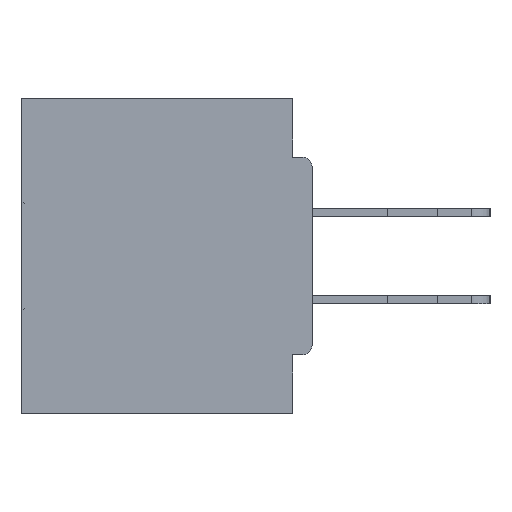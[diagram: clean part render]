
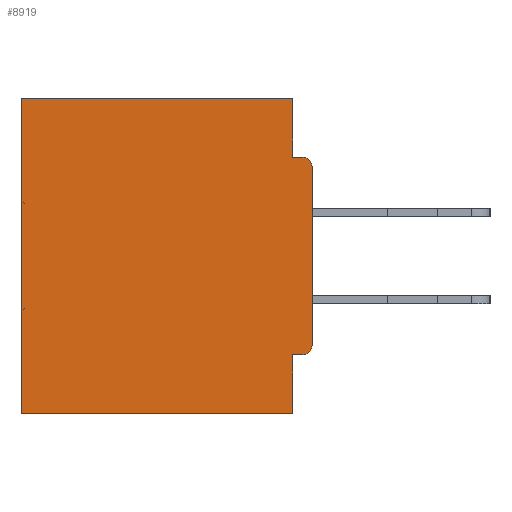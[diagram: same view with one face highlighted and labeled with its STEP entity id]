
A CAD part, left-side view. The second image highlights one B-rep face of the part: STEP entity #8919.
In plain terms, the highlighted planar face has unit normal (-1, 0, 0).
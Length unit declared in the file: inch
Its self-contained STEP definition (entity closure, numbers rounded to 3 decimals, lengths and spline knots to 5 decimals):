
#86 = DIRECTION ( 'NONE',  ( 0., 0., -1. ) ) ;
#171 = VERTEX_POINT ( 'NONE', #35271 ) ;
#204 = CARTESIAN_POINT ( 'NONE',  ( 0.298, 0.031, -0.5 ) ) ;
#538 = PLANE ( 'NONE',  #35679 ) ;
#1322 = EDGE_CURVE ( 'NONE', #26127, #38626, #14939, .T. ) ;
#1695 = CARTESIAN_POINT ( 'NONE',  ( 0.298, 0.015, -0.3915 ) ) ;
#2150 = CARTESIAN_POINT ( 'NONE',  ( 0.298, 0.015, -0.4065 ) ) ;
#3239 = CARTESIAN_POINT ( 'NONE',  ( 0.298, 0.031, -0.5 ) ) ;
#3848 = ORIENTED_EDGE ( 'NONE', *, *, #26362, .T. ) ;
#5564 = VERTEX_POINT ( 'NONE', #32588 ) ;
#6024 = CIRCLE ( 'NONE', #27586, 0.015 ) ;
#6758 = LINE ( 'NONE', #42754, #42551 ) ;
#7148 = ORIENTED_EDGE ( 'NONE', *, *, #35621, .F. ) ;
#7418 = DIRECTION ( 'NONE',  ( 0., 1., 0. ) ) ;
#8202 = VECTOR ( 'NONE', #37123, 39.37008 ) ;
#8390 = EDGE_CURVE ( 'NONE', #37002, #37179, #33414, .T. ) ;
#8805 = EDGE_LOOP ( 'NONE', ( #33632, #7148, #31541, #28815, #23127, #18778, #42385, #15322, #3848, #39202 ) ) ;
#8919 = ADVANCED_FACE ( 'NONE', ( #35030 ), #538, .F. ) ;
#9621 = VECTOR ( 'NONE', #30641, 39.37008 ) ;
#9954 = CARTESIAN_POINT ( 'NONE',  ( 0.298, 0.031, -0.5 ) ) ;
#10310 = CARTESIAN_POINT ( 'NONE',  ( 0.298, 0.031, -0.0935 ) ) ;
#10356 = CARTESIAN_POINT ( 'NONE',  ( 0.298, 0., 0. ) ) ;
#11106 = DIRECTION ( 'NONE',  ( 0., 0., -1. ) ) ;
#11273 = DIRECTION ( 'NONE',  ( 0., 1., 0. ) ) ;
#12420 = CARTESIAN_POINT ( 'NONE',  ( 0.298, 0., -0.3915 ) ) ;
#14620 = LINE ( 'NONE', #20014, #8202 ) ;
#14939 = CIRCLE ( 'NONE', #15940, 0.015 ) ;
#15322 = ORIENTED_EDGE ( 'NONE', *, *, #8390, .F. ) ;
#15940 = AXIS2_PLACEMENT_3D ( 'NONE', #19607, #43459, #26461 ) ;
#17151 = VECTOR ( 'NONE', #86, 39.37008 ) ;
#17632 = VECTOR ( 'NONE', #26953, 39.37008 ) ;
#17995 = CARTESIAN_POINT ( 'NONE',  ( 0.298, 0.031, 0. ) ) ;
#18615 = DIRECTION ( 'NONE',  ( 0., 0., -1. ) ) ;
#18778 = ORIENTED_EDGE ( 'NONE', *, *, #43936, .F. ) ;
#19500 = CARTESIAN_POINT ( 'NONE',  ( 0.298, 0., 0. ) ) ;
#19607 = CARTESIAN_POINT ( 'NONE',  ( 0.298, 0.015, -0.1085 ) ) ;
#20014 = CARTESIAN_POINT ( 'NONE',  ( 0.298, 0., -0.0935 ) ) ;
#20282 = LINE ( 'NONE', #19500, #17632 ) ;
#20614 = CARTESIAN_POINT ( 'NONE',  ( 0.298, 0., -0.5 ) ) ;
#20623 = EDGE_CURVE ( 'NONE', #26127, #36094, #25227, .T. ) ;
#21669 = EDGE_CURVE ( 'NONE', #33006, #5564, #20282, .T. ) ;
#22375 = DIRECTION ( 'NONE',  ( 0., 0., -1. ) ) ;
#23127 = ORIENTED_EDGE ( 'NONE', *, *, #39324, .T. ) ;
#23148 = LINE ( 'NONE', #20614, #28991 ) ;
#23327 = CARTESIAN_POINT ( 'NONE',  ( 0.298, 0., 0. ) ) ;
#25227 = LINE ( 'NONE', #23327, #40081 ) ;
#26127 = VERTEX_POINT ( 'NONE', #34726 ) ;
#26362 = EDGE_CURVE ( 'NONE', #37002, #36094, #6024, .T. ) ;
#26461 = DIRECTION ( 'NONE',  ( 0., 0., -1. ) ) ;
#26953 = DIRECTION ( 'NONE',  ( 0., 1., 0. ) ) ;
#27586 = AXIS2_PLACEMENT_3D ( 'NONE', #1695, #39011, #18615 ) ;
#28815 = ORIENTED_EDGE ( 'NONE', *, *, #21669, .T. ) ;
#28991 = VECTOR ( 'NONE', #7418, 39.37008 ) ;
#29258 = VERTEX_POINT ( 'NONE', #3239 ) ;
#29342 = CARTESIAN_POINT ( 'NONE',  ( 0.298, 0.015, -0.0935 ) ) ;
#30641 = DIRECTION ( 'NONE',  ( 0., 0., -1. ) ) ;
#31358 = EDGE_CURVE ( 'NONE', #37179, #29258, #32598, .T. ) ;
#31519 = CARTESIAN_POINT ( 'NONE',  ( 0.298, 0.031, -0.4065 ) ) ;
#31541 = ORIENTED_EDGE ( 'NONE', *, *, #36929, .F. ) ;
#32588 = CARTESIAN_POINT ( 'NONE',  ( 0.298, 0.46, 0. ) ) ;
#32598 = LINE ( 'NONE', #204, #9621 ) ;
#33006 = VERTEX_POINT ( 'NONE', #17995 ) ;
#33414 = LINE ( 'NONE', #34690, #43570 ) ;
#33632 = ORIENTED_EDGE ( 'NONE', *, *, #1322, .T. ) ;
#34690 = CARTESIAN_POINT ( 'NONE',  ( 0.298, 0., -0.4065 ) ) ;
#34726 = CARTESIAN_POINT ( 'NONE',  ( 0.298, 0., -0.1085 ) ) ;
#34829 = DIRECTION ( 'NONE',  ( 1., 0., 0. ) ) ;
#35030 = FACE_OUTER_BOUND ( 'NONE', #8805, .T. ) ;
#35271 = CARTESIAN_POINT ( 'NONE',  ( 0.298, 0.46, -0.5 ) ) ;
#35621 = EDGE_CURVE ( 'NONE', #42707, #38626, #14620, .T. ) ;
#35679 = AXIS2_PLACEMENT_3D ( 'NONE', #10356, #34829, #11106 ) ;
#36094 = VERTEX_POINT ( 'NONE', #12420 ) ;
#36929 = EDGE_CURVE ( 'NONE', #33006, #42707, #42790, .T. ) ;
#37002 = VERTEX_POINT ( 'NONE', #2150 ) ;
#37123 = DIRECTION ( 'NONE',  ( 0., -1., 0. ) ) ;
#37179 = VERTEX_POINT ( 'NONE', #31519 ) ;
#38626 = VERTEX_POINT ( 'NONE', #29342 ) ;
#39011 = DIRECTION ( 'NONE',  ( -1., 0., 0. ) ) ;
#39202 = ORIENTED_EDGE ( 'NONE', *, *, #20623, .F. ) ;
#39324 = EDGE_CURVE ( 'NONE', #5564, #171, #6758, .T. ) ;
#40081 = VECTOR ( 'NONE', #44164, 39.37008 ) ;
#42385 = ORIENTED_EDGE ( 'NONE', *, *, #31358, .F. ) ;
#42551 = VECTOR ( 'NONE', #22375, 39.37008 ) ;
#42707 = VERTEX_POINT ( 'NONE', #10310 ) ;
#42754 = CARTESIAN_POINT ( 'NONE',  ( 0.298, 0.46, 0. ) ) ;
#42790 = LINE ( 'NONE', #9954, #17151 ) ;
#43459 = DIRECTION ( 'NONE',  ( -1., 0., 0. ) ) ;
#43570 = VECTOR ( 'NONE', #11273, 39.37008 ) ;
#43936 = EDGE_CURVE ( 'NONE', #29258, #171, #23148, .T. ) ;
#44164 = DIRECTION ( 'NONE',  ( 0., 0., -1. ) ) ;
